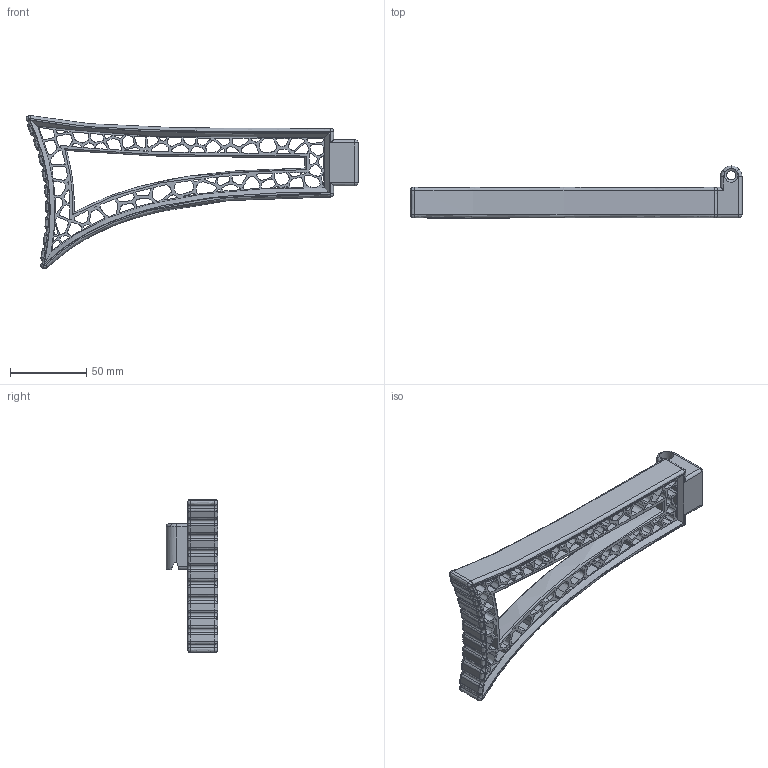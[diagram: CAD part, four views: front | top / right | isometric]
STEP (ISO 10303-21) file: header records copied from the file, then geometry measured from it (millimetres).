
FILE_DESCRIPTION(/* description */ (''),/* implementation_level */ '2;1');
FILE_NAME(/* name */ 'sharktail stock.step',/* time_stamp */ '2021-09-02T19:32:38-05:00',/* author */ (''),/* organization */ (''),/* preprocessor_version */ 'ST-DEVELOPER v18.1',/* originating_system */ 'Autodesk Translation Framework v10.10.0.1391',/* authorisation */ '');
FILE_SCHEMA (('AUTOMOTIVE_DESIGN { 1 0 10303 214 3 1 1 }'));
Length unit declared in the file: millimetre
Products named in the file (1): sharktail brace
Bounding box: 217.28 x 34 x 100.18 mm (x, y, z)
Volume: 103631.9 mm3; surface area: 57579.2 mm2
Topology: 1 solids, 1 shells, 654 faces, 1793 edges, 1135 vertices
Faces by surface type: bspline 501, sphere 46, plane 45, cylinder 36, torus 25, cone 1
Full cylindrical faces by diameter (mm): 6 x1, 9 x1, 11.2 x1
Entity records: 27134 total; most frequent: CARTESIAN_POINT 14602, ORIENTED_EDGE 3578, EDGE_CURVE 1789, DIRECTION 1350, VERTEX_POINT 1135, EDGE_LOOP 828, FACE_OUTER_BOUND 654, ADVANCED_FACE 654
